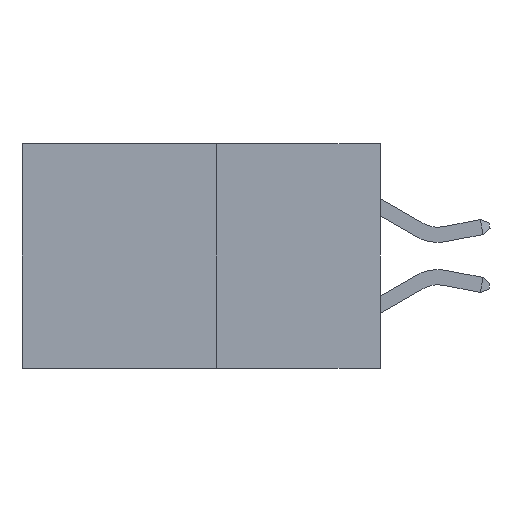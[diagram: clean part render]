
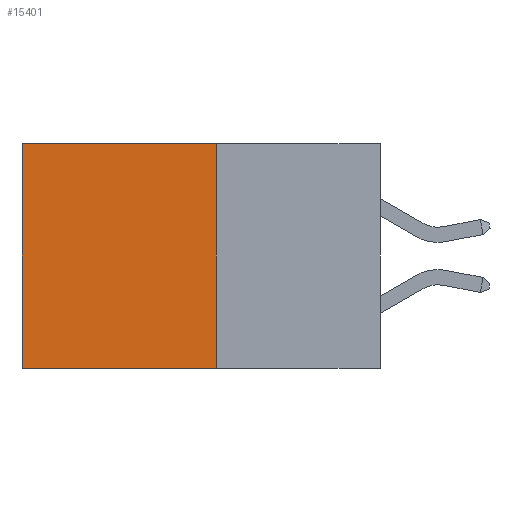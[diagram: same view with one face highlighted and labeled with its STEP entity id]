
A CAD part, left-side view. The second image highlights one B-rep face of the part: STEP entity #15401.
In plain terms, the highlighted planar face has unit normal (-1, 0, 0).
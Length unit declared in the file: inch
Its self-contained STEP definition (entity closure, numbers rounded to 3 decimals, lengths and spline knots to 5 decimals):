
#78 = FACE_OUTER_BOUND ( 'NONE', #8103, .T. ) ;
#295 = VECTOR ( 'NONE', #1164, 39.37008 ) ;
#606 = VERTEX_POINT ( 'NONE', #7756 ) ;
#1053 = DIRECTION ( 'NONE',  ( 1., 0., 0. ) ) ;
#1164 = DIRECTION ( 'NONE',  ( 0., 1., 0. ) ) ;
#1823 = EDGE_CURVE ( 'NONE', #2317, #606, #9783, .T. ) ;
#2317 = VERTEX_POINT ( 'NONE', #16681 ) ;
#2979 = DIRECTION ( 'NONE',  ( 0., 1., 0. ) ) ;
#3734 = VECTOR ( 'NONE', #7402, 39.37008 ) ;
#4017 = ORIENTED_EDGE ( 'NONE', *, *, #18761, .F. ) ;
#4495 = LINE ( 'NONE', #17762, #295 ) ;
#4541 = CARTESIAN_POINT ( 'NONE',  ( 0.277, 0.59, -0.37 ) ) ;
#5118 = ORIENTED_EDGE ( 'NONE', *, *, #18919, .F. ) ;
#7251 = ORIENTED_EDGE ( 'NONE', *, *, #1823, .T. ) ;
#7287 = CARTESIAN_POINT ( 'NONE',  ( 0.277, 0.27, -0.37 ) ) ;
#7402 = DIRECTION ( 'NONE',  ( 0., 0., -1. ) ) ;
#7589 = VERTEX_POINT ( 'NONE', #11598 ) ;
#7756 = CARTESIAN_POINT ( 'NONE',  ( 0.277, 0.59, -0.37 ) ) ;
#8103 = EDGE_LOOP ( 'NONE', ( #7251, #5118, #4017, #18628 ) ) ;
#9783 = LINE ( 'NONE', #4541, #13238 ) ;
#10026 = LINE ( 'NONE', #13642, #17779 ) ;
#11409 = LINE ( 'NONE', #17765, #3734 ) ;
#11598 = CARTESIAN_POINT ( 'NONE',  ( 0.277, 0.27, -0.37 ) ) ;
#11887 = DIRECTION ( 'NONE',  ( 0., 0., -1. ) ) ;
#12481 = VERTEX_POINT ( 'NONE', #12551 ) ;
#12551 = CARTESIAN_POINT ( 'NONE',  ( 0.277, 0.27, 0. ) ) ;
#13238 = VECTOR ( 'NONE', #15426, 39.37008 ) ;
#13642 = CARTESIAN_POINT ( 'NONE',  ( 0.277, 0.27, -0.37 ) ) ;
#15401 = ADVANCED_FACE ( 'NONE', ( #78 ), #17650, .F. ) ;
#15426 = DIRECTION ( 'NONE',  ( 0., 0., -1. ) ) ;
#16355 = EDGE_CURVE ( 'NONE', #12481, #2317, #4495, .T. ) ;
#16681 = CARTESIAN_POINT ( 'NONE',  ( 0.277, 0.59, 0. ) ) ;
#16758 = AXIS2_PLACEMENT_3D ( 'NONE', #7287, #1053, #11887 ) ;
#17650 = PLANE ( 'NONE',  #16758 ) ;
#17762 = CARTESIAN_POINT ( 'NONE',  ( 0.277, 0.27, 0. ) ) ;
#17765 = CARTESIAN_POINT ( 'NONE',  ( 0.277, 0.27, -0.37 ) ) ;
#17779 = VECTOR ( 'NONE', #2979, 39.37008 ) ;
#18628 = ORIENTED_EDGE ( 'NONE', *, *, #16355, .T. ) ;
#18761 = EDGE_CURVE ( 'NONE', #12481, #7589, #11409, .T. ) ;
#18919 = EDGE_CURVE ( 'NONE', #7589, #606, #10026, .T. ) ;
